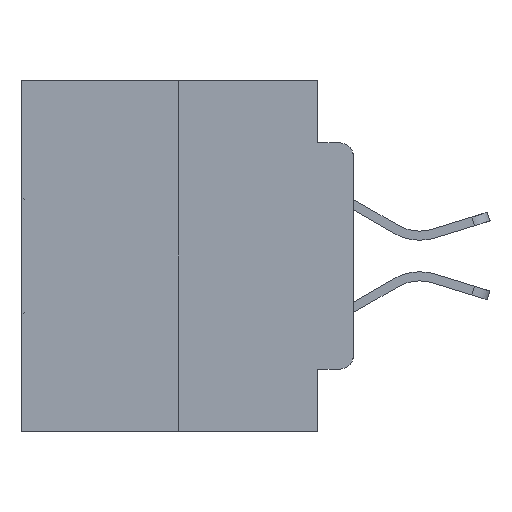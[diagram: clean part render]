
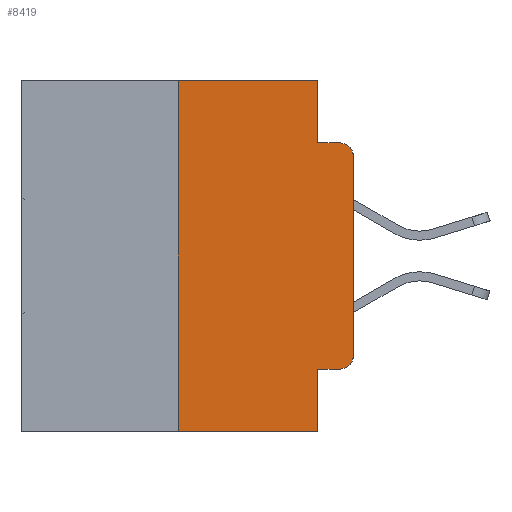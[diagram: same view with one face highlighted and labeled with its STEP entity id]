
A CAD part, left-side view. The second image highlights one B-rep face of the part: STEP entity #8419.
In plain terms, the highlighted planar face has unit normal (-1, 0, 0).
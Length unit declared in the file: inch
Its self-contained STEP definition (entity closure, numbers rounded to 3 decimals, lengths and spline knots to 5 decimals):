
#392 = ORIENTED_EDGE ( 'NONE', *, *, #26810, .F. ) ;
#451 = CARTESIAN_POINT ( 'NONE',  ( 0., 0., 0. ) ) ;
#737 = EDGE_CURVE ( 'NONE', #1242, #4305, #22520, .T. ) ;
#995 = VECTOR ( 'NONE', #28961, 39.37008 ) ;
#1242 = VERTEX_POINT ( 'NONE', #19391 ) ;
#1350 = EDGE_CURVE ( 'NONE', #3105, #1242, #1964, .T. ) ;
#1809 = CARTESIAN_POINT ( 'NONE',  ( 0., 0.02, -0.0885 ) ) ;
#1964 = CIRCLE ( 'NONE', #29470, 0.02 ) ;
#2447 = CARTESIAN_POINT ( 'NONE',  ( 0., 0.473, 0. ) ) ;
#2651 = DIRECTION ( 'NONE',  ( 0., 0., -1. ) ) ;
#2823 = VERTEX_POINT ( 'NONE', #12790 ) ;
#3048 = EDGE_CURVE ( 'NONE', #4677, #3105, #7328, .T. ) ;
#3105 = VERTEX_POINT ( 'NONE', #7219 ) ;
#3297 = EDGE_CURVE ( 'NONE', #15765, #20317, #6936, .T. ) ;
#3508 = VECTOR ( 'NONE', #19232, 39.37008 ) ;
#3590 = VECTOR ( 'NONE', #5713, 39.37008 ) ;
#4081 = CIRCLE ( 'NONE', #12123, 0.02 ) ;
#4305 = VERTEX_POINT ( 'NONE', #15723 ) ;
#4343 = ORIENTED_EDGE ( 'NONE', *, *, #3297, .T. ) ;
#4677 = VERTEX_POINT ( 'NONE', #6421 ) ;
#5713 = DIRECTION ( 'NONE',  ( 0., 0., 1. ) ) ;
#6241 = DIRECTION ( 'NONE',  ( 0., -1., 0. ) ) ;
#6421 = CARTESIAN_POINT ( 'NONE',  ( 0., 0.051, -0.4115 ) ) ;
#6579 = LINE ( 'NONE', #23597, #24534 ) ;
#6936 = LINE ( 'NONE', #7741, #18778 ) ;
#7219 = CARTESIAN_POINT ( 'NONE',  ( 0., 0.02, -0.4115 ) ) ;
#7328 = LINE ( 'NONE', #9442, #25927 ) ;
#7741 = CARTESIAN_POINT ( 'NONE',  ( 0., 0.473, -0.5 ) ) ;
#7750 = CARTESIAN_POINT ( 'NONE',  ( 0., 0.473, 0. ) ) ;
#7810 = DIRECTION ( 'NONE',  ( 0., 0., 1. ) ) ;
#8194 = ORIENTED_EDGE ( 'NONE', *, *, #22199, .F. ) ;
#8419 = ADVANCED_FACE ( 'NONE', ( #10699 ), #26453, .F. ) ;
#8561 = VERTEX_POINT ( 'NONE', #24760 ) ;
#8746 = VECTOR ( 'NONE', #7810, 39.37008 ) ;
#9129 = DIRECTION ( 'NONE',  ( 0., -1., 0. ) ) ;
#9283 = DIRECTION ( 'NONE',  ( 0., 0., -1. ) ) ;
#9337 = ORIENTED_EDGE ( 'NONE', *, *, #14463, .F. ) ;
#9442 = CARTESIAN_POINT ( 'NONE',  ( 0., 0.051, -0.4115 ) ) ;
#9671 = EDGE_CURVE ( 'NONE', #4677, #20317, #19756, .T. ) ;
#10699 = FACE_OUTER_BOUND ( 'NONE', #18664, .T. ) ;
#11534 = VERTEX_POINT ( 'NONE', #1809 ) ;
#12123 = AXIS2_PLACEMENT_3D ( 'NONE', #12667, #28719, #15023 ) ;
#12360 = ORIENTED_EDGE ( 'NONE', *, *, #3048, .T. ) ;
#12667 = CARTESIAN_POINT ( 'NONE',  ( 0., 0.02, -0.1085 ) ) ;
#12790 = CARTESIAN_POINT ( 'NONE',  ( 0., 0.051, 0. ) ) ;
#13595 = VECTOR ( 'NONE', #9283, 39.37008 ) ;
#14463 = EDGE_CURVE ( 'NONE', #15765, #8561, #26539, .T. ) ;
#15023 = DIRECTION ( 'NONE',  ( 0., 0., -1. ) ) ;
#15058 = DIRECTION ( 'NONE',  ( 0., 0., -1. ) ) ;
#15288 = ORIENTED_EDGE ( 'NONE', *, *, #1350, .T. ) ;
#15723 = CARTESIAN_POINT ( 'NONE',  ( 0., 0., -0.1085 ) ) ;
#15765 = VERTEX_POINT ( 'NONE', #24829 ) ;
#16653 = DIRECTION ( 'NONE',  ( -1., 0., 0. ) ) ;
#16801 = AXIS2_PLACEMENT_3D ( 'NONE', #7750, #28748, #15058 ) ;
#16888 = CARTESIAN_POINT ( 'NONE',  ( 0., 0.02, -0.3915 ) ) ;
#17052 = ORIENTED_EDGE ( 'NONE', *, *, #737, .T. ) ;
#18500 = ORIENTED_EDGE ( 'NONE', *, *, #29781, .T. ) ;
#18627 = CARTESIAN_POINT ( 'NONE',  ( 0., 0.051, 0. ) ) ;
#18664 = EDGE_LOOP ( 'NONE', ( #17052, #18500, #26010, #8194, #392, #9337, #4343, #29938, #12360, #15288 ) ) ;
#18778 = VECTOR ( 'NONE', #9129, 39.37008 ) ;
#19232 = DIRECTION ( 'NONE',  ( 0., -1., 0. ) ) ;
#19391 = CARTESIAN_POINT ( 'NONE',  ( 0., 0., -0.3915 ) ) ;
#19552 = CARTESIAN_POINT ( 'NONE',  ( 0., 0.25, 0. ) ) ;
#19756 = LINE ( 'NONE', #18627, #13595 ) ;
#20145 = LINE ( 'NONE', #26674, #995 ) ;
#20317 = VERTEX_POINT ( 'NONE', #25590 ) ;
#22199 = EDGE_CURVE ( 'NONE', #2823, #29677, #6579, .T. ) ;
#22520 = LINE ( 'NONE', #451, #3590 ) ;
#23597 = CARTESIAN_POINT ( 'NONE',  ( 0., 0.051, 0. ) ) ;
#23711 = EDGE_CURVE ( 'NONE', #29677, #11534, #20145, .T. ) ;
#24534 = VECTOR ( 'NONE', #25862, 39.37008 ) ;
#24760 = CARTESIAN_POINT ( 'NONE',  ( 0., 0.25, 0. ) ) ;
#24829 = CARTESIAN_POINT ( 'NONE',  ( 0., 0.25, -0.5 ) ) ;
#25590 = CARTESIAN_POINT ( 'NONE',  ( 0., 0.051, -0.5 ) ) ;
#25862 = DIRECTION ( 'NONE',  ( 0., 0., -1. ) ) ;
#25927 = VECTOR ( 'NONE', #6241, 39.37008 ) ;
#26010 = ORIENTED_EDGE ( 'NONE', *, *, #23711, .F. ) ;
#26453 = PLANE ( 'NONE',  #16801 ) ;
#26539 = LINE ( 'NONE', #19552, #8746 ) ;
#26674 = CARTESIAN_POINT ( 'NONE',  ( 0., 0.051, -0.0885 ) ) ;
#26810 = EDGE_CURVE ( 'NONE', #8561, #2823, #28493, .T. ) ;
#28136 = CARTESIAN_POINT ( 'NONE',  ( 0., 0.051, -0.0885 ) ) ;
#28493 = LINE ( 'NONE', #2447, #3508 ) ;
#28719 = DIRECTION ( 'NONE',  ( -1., 0., 0. ) ) ;
#28748 = DIRECTION ( 'NONE',  ( 1., 0., 0. ) ) ;
#28961 = DIRECTION ( 'NONE',  ( 0., -1., 0. ) ) ;
#29470 = AXIS2_PLACEMENT_3D ( 'NONE', #16888, #16653, #2651 ) ;
#29677 = VERTEX_POINT ( 'NONE', #28136 ) ;
#29781 = EDGE_CURVE ( 'NONE', #4305, #11534, #4081, .T. ) ;
#29938 = ORIENTED_EDGE ( 'NONE', *, *, #9671, .F. ) ;
